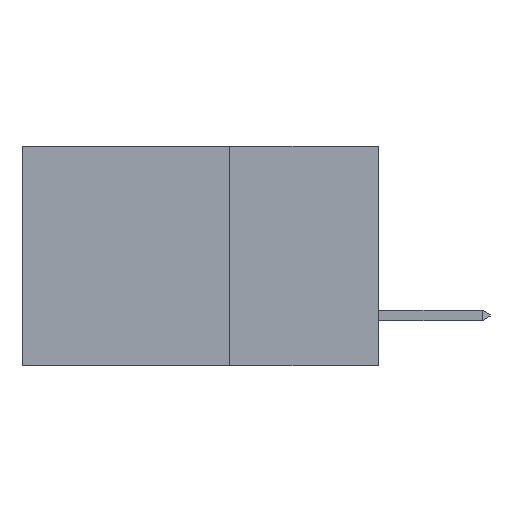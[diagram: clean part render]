
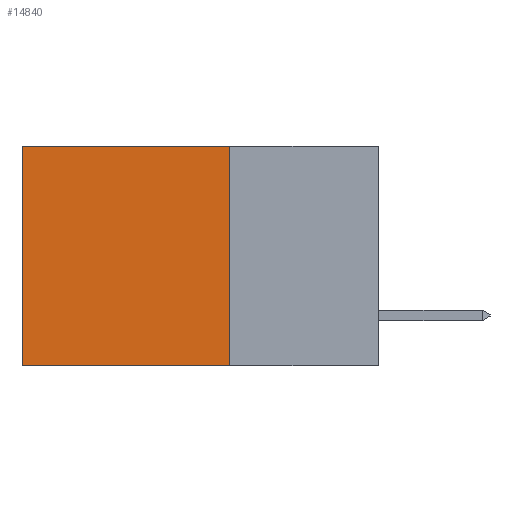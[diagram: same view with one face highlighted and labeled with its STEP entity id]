
A CAD part, left-side view. The second image highlights one B-rep face of the part: STEP entity #14840.
In plain terms, the highlighted planar face has unit normal (-1, 0, 0).
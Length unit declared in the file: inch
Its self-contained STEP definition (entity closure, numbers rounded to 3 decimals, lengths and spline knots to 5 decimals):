
#219 = FACE_OUTER_BOUND ( 'NONE', #12559, .T. ) ;
#1120 = CARTESIAN_POINT ( 'NONE',  ( 0.2615, 0.25, 0. ) ) ;
#1857 = LINE ( 'NONE', #9069, #14698 ) ;
#1888 = EDGE_CURVE ( 'NONE', #15279, #5405, #1857, .T. ) ;
#2031 = ORIENTED_EDGE ( 'NONE', *, *, #1888, .T. ) ;
#2137 = EDGE_CURVE ( 'NONE', #13424, #5405, #14863, .T. ) ;
#2554 = ORIENTED_EDGE ( 'NONE', *, *, #2137, .F. ) ;
#2995 = CARTESIAN_POINT ( 'NONE',  ( 0.2615, 0.25, 0. ) ) ;
#3803 = DIRECTION ( 'NONE',  ( 1., 0., 0. ) ) ;
#3972 = ORIENTED_EDGE ( 'NONE', *, *, #6743, .F. ) ;
#4933 = VERTEX_POINT ( 'NONE', #1120 ) ;
#5405 = VERTEX_POINT ( 'NONE', #15204 ) ;
#5803 = AXIS2_PLACEMENT_3D ( 'NONE', #8845, #3803, #12543 ) ;
#6743 = EDGE_CURVE ( 'NONE', #4933, #13424, #9946, .T. ) ;
#7455 = DIRECTION ( 'NONE',  ( 0., 0., -1. ) ) ;
#7557 = CARTESIAN_POINT ( 'NONE',  ( 0.2615, 0.25, -0.37 ) ) ;
#8401 = VECTOR ( 'NONE', #13442, 39.37008 ) ;
#8845 = CARTESIAN_POINT ( 'NONE',  ( 0.2615, 0.25, -0.37 ) ) ;
#8853 = DIRECTION ( 'NONE',  ( 0., 0., -1. ) ) ;
#9069 = CARTESIAN_POINT ( 'NONE',  ( 0.2615, 0.6, -0.37 ) ) ;
#9326 = ORIENTED_EDGE ( 'NONE', *, *, #9458, .T. ) ;
#9458 = EDGE_CURVE ( 'NONE', #4933, #15279, #15130, .T. ) ;
#9946 = LINE ( 'NONE', #7557, #12804 ) ;
#11331 = PLANE ( 'NONE',  #5803 ) ;
#11952 = VECTOR ( 'NONE', #14187, 39.37008 ) ;
#12543 = DIRECTION ( 'NONE',  ( 0., 0., -1. ) ) ;
#12559 = EDGE_LOOP ( 'NONE', ( #2031, #2554, #3972, #9326 ) ) ;
#12804 = VECTOR ( 'NONE', #7455, 39.37008 ) ;
#13424 = VERTEX_POINT ( 'NONE', #13554 ) ;
#13442 = DIRECTION ( 'NONE',  ( 0., 1., 0. ) ) ;
#13554 = CARTESIAN_POINT ( 'NONE',  ( 0.2615, 0.25, -0.37 ) ) ;
#13603 = CARTESIAN_POINT ( 'NONE',  ( 0.2615, 0.25, -0.37 ) ) ;
#14187 = DIRECTION ( 'NONE',  ( 0., 1., 0. ) ) ;
#14420 = CARTESIAN_POINT ( 'NONE',  ( 0.2615, 0.6, 0. ) ) ;
#14698 = VECTOR ( 'NONE', #8853, 39.37008 ) ;
#14840 = ADVANCED_FACE ( 'NONE', ( #219 ), #11331, .F. ) ;
#14863 = LINE ( 'NONE', #13603, #8401 ) ;
#15130 = LINE ( 'NONE', #2995, #11952 ) ;
#15204 = CARTESIAN_POINT ( 'NONE',  ( 0.2615, 0.6, -0.37 ) ) ;
#15279 = VERTEX_POINT ( 'NONE', #14420 ) ;
